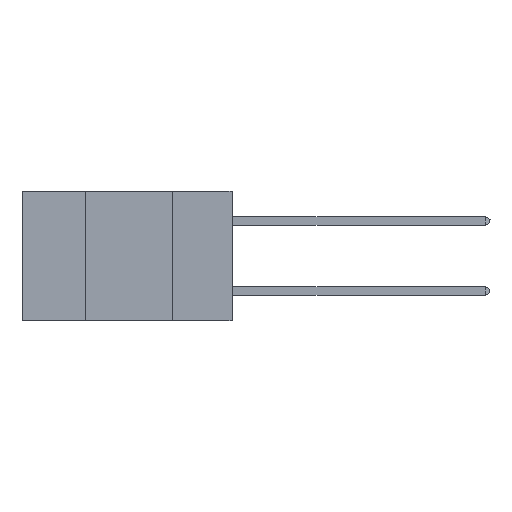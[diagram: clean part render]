
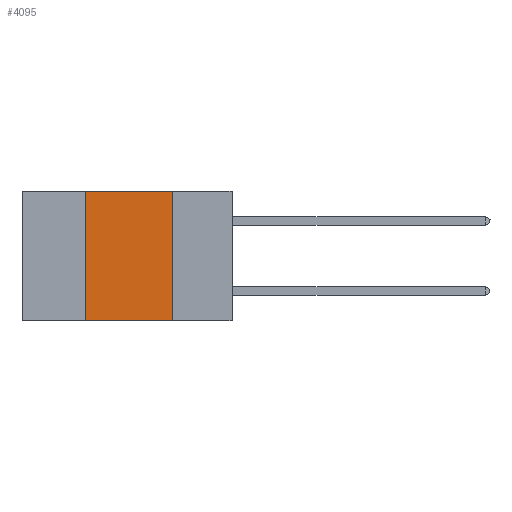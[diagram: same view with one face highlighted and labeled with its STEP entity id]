
A CAD part, left-side view. The second image highlights one B-rep face of the part: STEP entity #4095.
In plain terms, the highlighted planar face has unit normal (-1, 0, 0).
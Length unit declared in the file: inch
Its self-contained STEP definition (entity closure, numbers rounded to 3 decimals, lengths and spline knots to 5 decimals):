
#222 = CARTESIAN_POINT ( 'NONE',  ( 0., 0.17, -0.37 ) ) ;
#227 = EDGE_LOOP ( 'NONE', ( #6278, #10405, #8360, #10683 ) ) ;
#645 = CARTESIAN_POINT ( 'NONE',  ( 0., 0.42, 0. ) ) ;
#762 = VERTEX_POINT ( 'NONE', #645 ) ;
#1069 = VERTEX_POINT ( 'NONE', #9188 ) ;
#1185 = PLANE ( 'NONE',  #5521 ) ;
#1748 = CARTESIAN_POINT ( 'NONE',  ( 0., 0.17, 0. ) ) ;
#2080 = VECTOR ( 'NONE', #9507, 39.37008 ) ;
#2083 = DIRECTION ( 'NONE',  ( 0., 0., -1. ) ) ;
#3138 = VECTOR ( 'NONE', #3435, 39.37008 ) ;
#3252 = CARTESIAN_POINT ( 'NONE',  ( 0., 0.6, 0. ) ) ;
#3435 = DIRECTION ( 'NONE',  ( 0., -1., 0. ) ) ;
#4031 = DIRECTION ( 'NONE',  ( 1., 0., 0. ) ) ;
#4095 = ADVANCED_FACE ( 'NONE', ( #9015 ), #1185, .F. ) ;
#4584 = CARTESIAN_POINT ( 'NONE',  ( 0., 0.6, -0.37 ) ) ;
#4698 = EDGE_CURVE ( 'NONE', #762, #1069, #12262, .T. ) ;
#5290 = EDGE_CURVE ( 'NONE', #7923, #762, #6803, .T. ) ;
#5486 = VERTEX_POINT ( 'NONE', #222 ) ;
#5521 = AXIS2_PLACEMENT_3D ( 'NONE', #11761, #4031, #2083 ) ;
#5544 = LINE ( 'NONE', #4584, #2080 ) ;
#5609 = VECTOR ( 'NONE', #10672, 39.37008 ) ;
#6278 = ORIENTED_EDGE ( 'NONE', *, *, #11594, .F. ) ;
#6676 = CARTESIAN_POINT ( 'NONE',  ( 0., 0.42, 0. ) ) ;
#6803 = LINE ( 'NONE', #6676, #5609 ) ;
#7923 = VERTEX_POINT ( 'NONE', #11050 ) ;
#8360 = ORIENTED_EDGE ( 'NONE', *, *, #5290, .F. ) ;
#9015 = FACE_OUTER_BOUND ( 'NONE', #227, .T. ) ;
#9188 = CARTESIAN_POINT ( 'NONE',  ( 0., 0.17, 0. ) ) ;
#9507 = DIRECTION ( 'NONE',  ( 0., -1., 0. ) ) ;
#9649 = DIRECTION ( 'NONE',  ( 0., 0., -1. ) ) ;
#10405 = ORIENTED_EDGE ( 'NONE', *, *, #4698, .F. ) ;
#10602 = LINE ( 'NONE', #1748, #11144 ) ;
#10672 = DIRECTION ( 'NONE',  ( 0., 0., 1. ) ) ;
#10683 = ORIENTED_EDGE ( 'NONE', *, *, #10894, .T. ) ;
#10894 = EDGE_CURVE ( 'NONE', #7923, #5486, #5544, .T. ) ;
#11050 = CARTESIAN_POINT ( 'NONE',  ( 0., 0.42, -0.37 ) ) ;
#11144 = VECTOR ( 'NONE', #9649, 39.37008 ) ;
#11594 = EDGE_CURVE ( 'NONE', #1069, #5486, #10602, .T. ) ;
#11761 = CARTESIAN_POINT ( 'NONE',  ( 0., 0.6, 0. ) ) ;
#12262 = LINE ( 'NONE', #3252, #3138 ) ;
